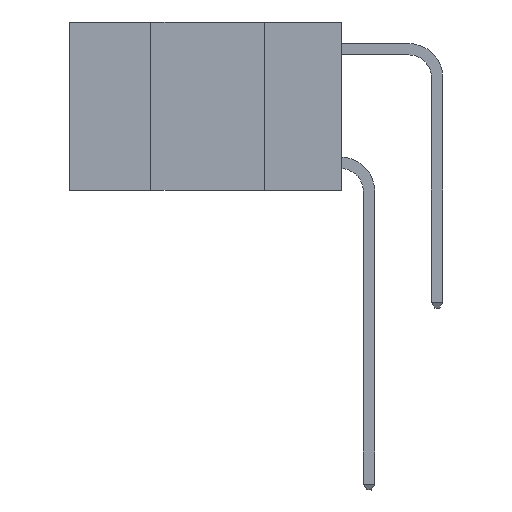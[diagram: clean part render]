
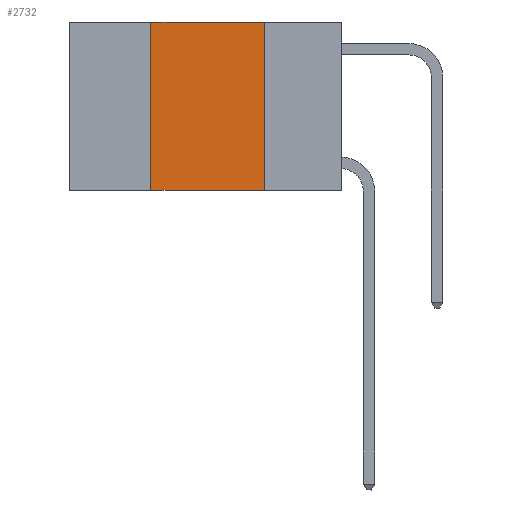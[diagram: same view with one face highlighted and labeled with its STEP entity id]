
A CAD part, left-side view. The second image highlights one B-rep face of the part: STEP entity #2732.
In plain terms, the highlighted planar face has unit normal (-1, 0, 0).
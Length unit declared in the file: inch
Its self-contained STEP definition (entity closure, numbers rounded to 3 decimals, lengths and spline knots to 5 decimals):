
#166 = ORIENTED_EDGE ( 'NONE', *, *, #4622, .T. ) ;
#2567 = LINE ( 'NONE', #4312, #12623 ) ;
#2732 = ADVANCED_FACE ( 'NONE', ( #11643 ), #9565, .F. ) ;
#3031 = CARTESIAN_POINT ( 'NONE',  ( 0., 0.6, 0. ) ) ;
#3590 = VECTOR ( 'NONE', #5060, 39.37008 ) ;
#4312 = CARTESIAN_POINT ( 'NONE',  ( 0., 0.6, -0.37 ) ) ;
#4353 = DIRECTION ( 'NONE',  ( 0., 0., -1. ) ) ;
#4622 = EDGE_CURVE ( 'NONE', #15979, #4632, #2567, .T. ) ;
#4632 = VERTEX_POINT ( 'NONE', #8267 ) ;
#5060 = DIRECTION ( 'NONE',  ( 0., -1., 0. ) ) ;
#5620 = DIRECTION ( 'NONE',  ( 0., -1., 0. ) ) ;
#5774 = VECTOR ( 'NONE', #13295, 39.37008 ) ;
#6022 = ORIENTED_EDGE ( 'NONE', *, *, #16913, .F. ) ;
#6126 = CARTESIAN_POINT ( 'NONE',  ( 0., 0.42, -0.37 ) ) ;
#6177 = LINE ( 'NONE', #14435, #9669 ) ;
#6764 = AXIS2_PLACEMENT_3D ( 'NONE', #3031, #12219, #4353 ) ;
#7005 = LINE ( 'NONE', #9392, #5774 ) ;
#7623 = CARTESIAN_POINT ( 'NONE',  ( 0., 0.42, 0. ) ) ;
#7883 = VERTEX_POINT ( 'NONE', #7623 ) ;
#8267 = CARTESIAN_POINT ( 'NONE',  ( 0., 0.17, -0.37 ) ) ;
#8977 = CARTESIAN_POINT ( 'NONE',  ( 0., 0.6, 0. ) ) ;
#9348 = EDGE_CURVE ( 'NONE', #15979, #7883, #7005, .T. ) ;
#9392 = CARTESIAN_POINT ( 'NONE',  ( 0., 0.42, 0. ) ) ;
#9565 = PLANE ( 'NONE',  #6764 ) ;
#9669 = VECTOR ( 'NONE', #10448, 39.37008 ) ;
#10448 = DIRECTION ( 'NONE',  ( 0., 0., -1. ) ) ;
#10994 = LINE ( 'NONE', #8977, #3590 ) ;
#11643 = FACE_OUTER_BOUND ( 'NONE', #12561, .T. ) ;
#12158 = CARTESIAN_POINT ( 'NONE',  ( 0., 0.17, 0. ) ) ;
#12219 = DIRECTION ( 'NONE',  ( 1., 0., 0. ) ) ;
#12561 = EDGE_LOOP ( 'NONE', ( #15769, #6022, #16500, #166 ) ) ;
#12623 = VECTOR ( 'NONE', #5620, 39.37008 ) ;
#13295 = DIRECTION ( 'NONE',  ( 0., 0., 1. ) ) ;
#13578 = EDGE_CURVE ( 'NONE', #14450, #4632, #6177, .T. ) ;
#14435 = CARTESIAN_POINT ( 'NONE',  ( 0., 0.17, 0. ) ) ;
#14450 = VERTEX_POINT ( 'NONE', #12158 ) ;
#15769 = ORIENTED_EDGE ( 'NONE', *, *, #13578, .F. ) ;
#15979 = VERTEX_POINT ( 'NONE', #6126 ) ;
#16500 = ORIENTED_EDGE ( 'NONE', *, *, #9348, .F. ) ;
#16913 = EDGE_CURVE ( 'NONE', #7883, #14450, #10994, .T. ) ;
